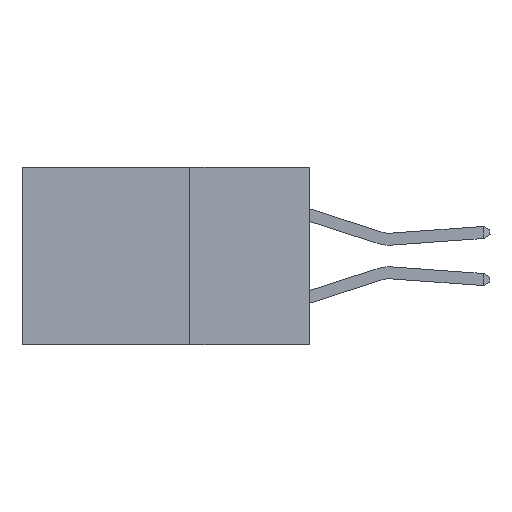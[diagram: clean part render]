
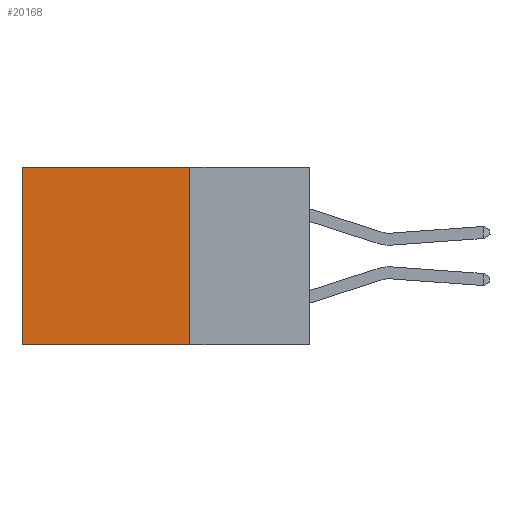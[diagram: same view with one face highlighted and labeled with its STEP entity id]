
A CAD part, left-side view. The second image highlights one B-rep face of the part: STEP entity #20168.
In plain terms, the highlighted planar face has unit normal (-1, 0, 0).
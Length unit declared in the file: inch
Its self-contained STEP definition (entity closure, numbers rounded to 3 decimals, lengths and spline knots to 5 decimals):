
#8 = DIRECTION ( 'NONE',  ( 1., 0., 0. ) ) ;
#884 = VECTOR ( 'NONE', #2803, 39.37008 ) ;
#1320 = CARTESIAN_POINT ( 'NONE',  ( 0.2615, 0.6, -0.37 ) ) ;
#1736 = VERTEX_POINT ( 'NONE', #22774 ) ;
#2103 = CARTESIAN_POINT ( 'NONE',  ( 0.2615, 0.25, 0. ) ) ;
#2803 = DIRECTION ( 'NONE',  ( 0., 1., 0. ) ) ;
#2945 = VECTOR ( 'NONE', #17860, 39.37008 ) ;
#3073 = VECTOR ( 'NONE', #6592, 39.37008 ) ;
#3869 = EDGE_LOOP ( 'NONE', ( #19506, #18238, #13477, #21812 ) ) ;
#4746 = LINE ( 'NONE', #1320, #3073 ) ;
#6506 = EDGE_CURVE ( 'NONE', #17268, #21833, #15906, .T. ) ;
#6592 = DIRECTION ( 'NONE',  ( 0., 0., -1. ) ) ;
#6727 = AXIS2_PLACEMENT_3D ( 'NONE', #9310, #8, #9553 ) ;
#7756 = DIRECTION ( 'NONE',  ( 0., 0., -1. ) ) ;
#9253 = CARTESIAN_POINT ( 'NONE',  ( 0.2615, 0.25, -0.37 ) ) ;
#9310 = CARTESIAN_POINT ( 'NONE',  ( 0.2615, 0.25, -0.37 ) ) ;
#9448 = CARTESIAN_POINT ( 'NONE',  ( 0.2615, 0.25, -0.37 ) ) ;
#9482 = VECTOR ( 'NONE', #7756, 39.37008 ) ;
#9553 = DIRECTION ( 'NONE',  ( 0., 0., -1. ) ) ;
#11029 = FACE_OUTER_BOUND ( 'NONE', #3869, .T. ) ;
#12177 = VERTEX_POINT ( 'NONE', #9448 ) ;
#13379 = LINE ( 'NONE', #9253, #9482 ) ;
#13477 = ORIENTED_EDGE ( 'NONE', *, *, #21205, .F. ) ;
#15906 = LINE ( 'NONE', #16145, #2945 ) ;
#16004 = EDGE_CURVE ( 'NONE', #21833, #1736, #4746, .T. ) ;
#16145 = CARTESIAN_POINT ( 'NONE',  ( 0.2615, 0.25, 0. ) ) ;
#16683 = PLANE ( 'NONE',  #6727 ) ;
#17268 = VERTEX_POINT ( 'NONE', #2103 ) ;
#17414 = CARTESIAN_POINT ( 'NONE',  ( 0.2615, 0.6, 0. ) ) ;
#17860 = DIRECTION ( 'NONE',  ( 0., 1., 0. ) ) ;
#18141 = LINE ( 'NONE', #20117, #884 ) ;
#18238 = ORIENTED_EDGE ( 'NONE', *, *, #22656, .F. ) ;
#19506 = ORIENTED_EDGE ( 'NONE', *, *, #16004, .T. ) ;
#20117 = CARTESIAN_POINT ( 'NONE',  ( 0.2615, 0.25, -0.37 ) ) ;
#20168 = ADVANCED_FACE ( 'NONE', ( #11029 ), #16683, .F. ) ;
#21205 = EDGE_CURVE ( 'NONE', #17268, #12177, #13379, .T. ) ;
#21812 = ORIENTED_EDGE ( 'NONE', *, *, #6506, .T. ) ;
#21833 = VERTEX_POINT ( 'NONE', #17414 ) ;
#22656 = EDGE_CURVE ( 'NONE', #12177, #1736, #18141, .T. ) ;
#22774 = CARTESIAN_POINT ( 'NONE',  ( 0.2615, 0.6, -0.37 ) ) ;
